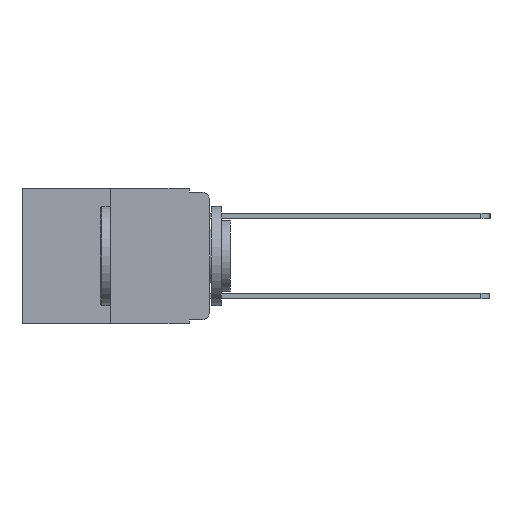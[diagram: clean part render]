
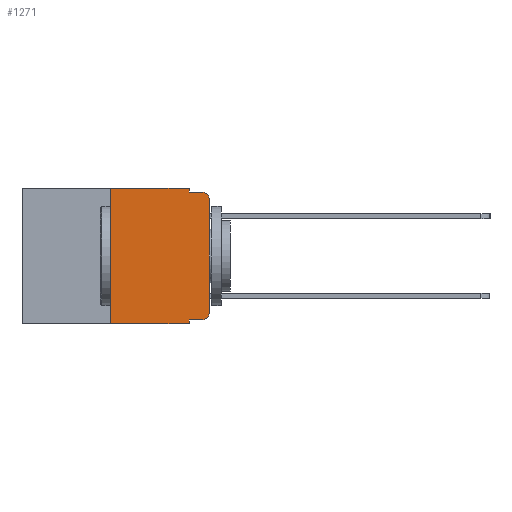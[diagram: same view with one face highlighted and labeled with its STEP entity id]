
A CAD part, left-side view. The second image highlights one B-rep face of the part: STEP entity #1271.
In plain terms, the highlighted planar face has unit normal (-1, 0, 0).
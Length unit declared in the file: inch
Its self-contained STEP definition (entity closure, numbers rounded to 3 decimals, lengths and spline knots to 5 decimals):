
#308 = EDGE_CURVE ( 'NONE', #2408, #4804, #10090, .T. ) ;
#591 = VECTOR ( 'NONE', #10418, 39.37008 ) ;
#597 = VECTOR ( 'NONE', #719, 39.37008 ) ;
#659 = CARTESIAN_POINT ( 'NONE',  ( 0., 0.051, -0.343 ) ) ;
#719 = DIRECTION ( 'NONE',  ( 0., -1., 0. ) ) ;
#885 = ORIENTED_EDGE ( 'NONE', *, *, #2423, .F. ) ;
#1020 = EDGE_CURVE ( 'NONE', #4604, #4832, #9267, .T. ) ;
#1263 = LINE ( 'NONE', #8847, #597 ) ;
#1271 = ADVANCED_FACE ( 'NONE', ( #5594 ), #4007, .F. ) ;
#1320 = ORIENTED_EDGE ( 'NONE', *, *, #3069, .T. ) ;
#1697 = AXIS2_PLACEMENT_3D ( 'NONE', #1999, #3964, #3365 ) ;
#1857 = ORIENTED_EDGE ( 'NONE', *, *, #3770, .T. ) ;
#1999 = CARTESIAN_POINT ( 'NONE',  ( 0., 0.473, 0. ) ) ;
#2014 = LINE ( 'NONE', #8562, #11561 ) ;
#2408 = VERTEX_POINT ( 'NONE', #3488 ) ;
#2423 = EDGE_CURVE ( 'NONE', #4832, #11954, #6471, .T. ) ;
#2637 = CARTESIAN_POINT ( 'NONE',  ( 0., 0.02, -0.313 ) ) ;
#2950 = CIRCLE ( 'NONE', #9568, 0.02 ) ;
#3069 = EDGE_CURVE ( 'NONE', #6651, #11954, #2950, .T. ) ;
#3234 = VERTEX_POINT ( 'NONE', #4795 ) ;
#3365 = DIRECTION ( 'NONE',  ( 0., 0., -1. ) ) ;
#3488 = CARTESIAN_POINT ( 'NONE',  ( 0., 0.25, -0.343 ) ) ;
#3621 = CARTESIAN_POINT ( 'NONE',  ( 0., 0., -0.03 ) ) ;
#3687 = DIRECTION ( 'NONE',  ( 0., 0., -1. ) ) ;
#3770 = EDGE_CURVE ( 'NONE', #4818, #6651, #2014, .T. ) ;
#3886 = CARTESIAN_POINT ( 'NONE',  ( 0., 0.051, -0.01 ) ) ;
#3943 = CARTESIAN_POINT ( 'NONE',  ( 0., 0.051, 0. ) ) ;
#3964 = DIRECTION ( 'NONE',  ( 1., 0., 0. ) ) ;
#4007 = PLANE ( 'NONE',  #1697 ) ;
#4137 = EDGE_LOOP ( 'NONE', ( #1857, #1320, #885, #5457, #5771, #5922, #5978, #6136, #9896, #6226 ) ) ;
#4522 = LINE ( 'NONE', #12113, #9439 ) ;
#4562 = CARTESIAN_POINT ( 'NONE',  ( 0., 0.051, -0.333 ) ) ;
#4604 = VERTEX_POINT ( 'NONE', #5710 ) ;
#4713 = CARTESIAN_POINT ( 'NONE',  ( 0., 0.02, -0.01 ) ) ;
#4795 = CARTESIAN_POINT ( 'NONE',  ( 0., 0.02, -0.333 ) ) ;
#4804 = VERTEX_POINT ( 'NONE', #8790 ) ;
#4818 = VERTEX_POINT ( 'NONE', #8829 ) ;
#4832 = VERTEX_POINT ( 'NONE', #3886 ) ;
#5307 = CARTESIAN_POINT ( 'NONE',  ( 0., 0.051, 0. ) ) ;
#5406 = VECTOR ( 'NONE', #9867, 39.37008 ) ;
#5457 = ORIENTED_EDGE ( 'NONE', *, *, #1020, .F. ) ;
#5594 = FACE_OUTER_BOUND ( 'NONE', #4137, .T. ) ;
#5710 = CARTESIAN_POINT ( 'NONE',  ( 0., 0.051, 0. ) ) ;
#5771 = ORIENTED_EDGE ( 'NONE', *, *, #7067, .F. ) ;
#5922 = ORIENTED_EDGE ( 'NONE', *, *, #308, .F. ) ;
#5978 = ORIENTED_EDGE ( 'NONE', *, *, #8241, .T. ) ;
#6136 = ORIENTED_EDGE ( 'NONE', *, *, #12474, .F. ) ;
#6226 = ORIENTED_EDGE ( 'NONE', *, *, #11238, .T. ) ;
#6471 = LINE ( 'NONE', #12088, #8794 ) ;
#6651 = VERTEX_POINT ( 'NONE', #3621 ) ;
#7067 = EDGE_CURVE ( 'NONE', #4804, #4604, #4522, .T. ) ;
#7423 = LINE ( 'NONE', #3943, #5406 ) ;
#7536 = AXIS2_PLACEMENT_3D ( 'NONE', #2637, #9604, #3687 ) ;
#7564 = DIRECTION ( 'NONE',  ( 0., -1., 0. ) ) ;
#8241 = EDGE_CURVE ( 'NONE', #2408, #8778, #1263, .T. ) ;
#8377 = DIRECTION ( 'NONE',  ( 0., -1., 0. ) ) ;
#8562 = CARTESIAN_POINT ( 'NONE',  ( 0., 0., 0. ) ) ;
#8576 = DIRECTION ( 'NONE',  ( 0., 0., 1. ) ) ;
#8778 = VERTEX_POINT ( 'NONE', #659 ) ;
#8790 = CARTESIAN_POINT ( 'NONE',  ( 0., 0.25, 0. ) ) ;
#8794 = VECTOR ( 'NONE', #7564, 39.37008 ) ;
#8829 = CARTESIAN_POINT ( 'NONE',  ( 0., 0., -0.313 ) ) ;
#8847 = CARTESIAN_POINT ( 'NONE',  ( 0., 0.473, -0.343 ) ) ;
#8852 = CARTESIAN_POINT ( 'NONE',  ( 0., 0.25, 0. ) ) ;
#9198 = DIRECTION ( 'NONE',  ( 0., 0., -1. ) ) ;
#9216 = DIRECTION ( 'NONE',  ( -1., 0., 0. ) ) ;
#9267 = LINE ( 'NONE', #5307, #11484 ) ;
#9301 = CARTESIAN_POINT ( 'NONE',  ( 0., 0.02, -0.03 ) ) ;
#9351 = DIRECTION ( 'NONE',  ( 0., 0., -1. ) ) ;
#9439 = VECTOR ( 'NONE', #8377, 39.37008 ) ;
#9495 = VERTEX_POINT ( 'NONE', #12569 ) ;
#9568 = AXIS2_PLACEMENT_3D ( 'NONE', #9301, #9216, #9198 ) ;
#9604 = DIRECTION ( 'NONE',  ( -1., 0., 0. ) ) ;
#9867 = DIRECTION ( 'NONE',  ( 0., 0., -1. ) ) ;
#9896 = ORIENTED_EDGE ( 'NONE', *, *, #11852, .T. ) ;
#10090 = LINE ( 'NONE', #8852, #12786 ) ;
#10418 = DIRECTION ( 'NONE',  ( 0., -1., 0. ) ) ;
#10587 = CIRCLE ( 'NONE', #7536, 0.02 ) ;
#10589 = DIRECTION ( 'NONE',  ( 0., 0., 1. ) ) ;
#11238 = EDGE_CURVE ( 'NONE', #3234, #4818, #10587, .T. ) ;
#11466 = LINE ( 'NONE', #4562, #591 ) ;
#11484 = VECTOR ( 'NONE', #9351, 39.37008 ) ;
#11561 = VECTOR ( 'NONE', #8576, 39.37008 ) ;
#11852 = EDGE_CURVE ( 'NONE', #9495, #3234, #11466, .T. ) ;
#11954 = VERTEX_POINT ( 'NONE', #4713 ) ;
#12088 = CARTESIAN_POINT ( 'NONE',  ( 0., 0.051, -0.01 ) ) ;
#12113 = CARTESIAN_POINT ( 'NONE',  ( 0., 0.473, 0. ) ) ;
#12474 = EDGE_CURVE ( 'NONE', #9495, #8778, #7423, .T. ) ;
#12569 = CARTESIAN_POINT ( 'NONE',  ( 0., 0.051, -0.333 ) ) ;
#12786 = VECTOR ( 'NONE', #10589, 39.37008 ) ;
